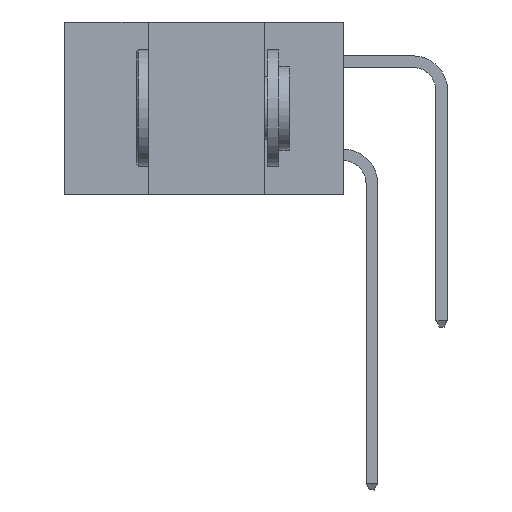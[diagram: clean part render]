
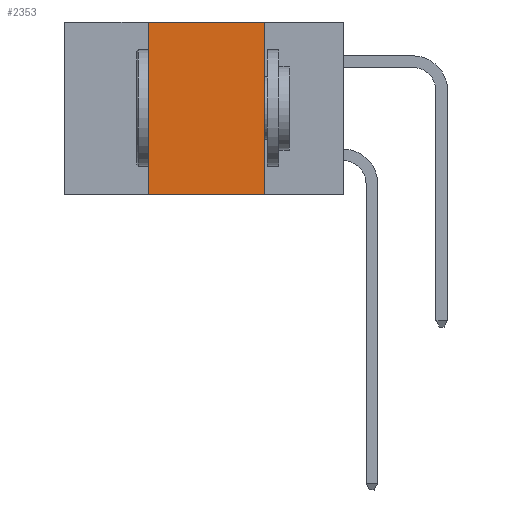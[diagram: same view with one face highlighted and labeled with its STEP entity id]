
A CAD part, left-side view. The second image highlights one B-rep face of the part: STEP entity #2353.
In plain terms, the highlighted planar face has unit normal (-1, 0, 0).
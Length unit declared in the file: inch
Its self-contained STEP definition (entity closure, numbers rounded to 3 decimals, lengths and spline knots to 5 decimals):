
#746 = VECTOR ( 'NONE', #16608, 39.37008 ) ;
#815 = CARTESIAN_POINT ( 'NONE',  ( 0., 0.6, 0. ) ) ;
#844 = CARTESIAN_POINT ( 'NONE',  ( 0., 0.17, 0. ) ) ;
#1459 = ORIENTED_EDGE ( 'NONE', *, *, #2229, .T. ) ;
#2229 = EDGE_CURVE ( 'NONE', #6645, #19244, #9526, .T. ) ;
#2277 = PLANE ( 'NONE',  #7809 ) ;
#2353 = ADVANCED_FACE ( 'NONE', ( #14612 ), #2277, .F. ) ;
#2810 = DIRECTION ( 'NONE',  ( 0., -1., 0. ) ) ;
#3383 = CARTESIAN_POINT ( 'NONE',  ( 0., 0.17, 0. ) ) ;
#3513 = CARTESIAN_POINT ( 'NONE',  ( 0., 0.42, 0. ) ) ;
#4089 = ORIENTED_EDGE ( 'NONE', *, *, #16455, .F. ) ;
#4369 = DIRECTION ( 'NONE',  ( 1., 0., 0. ) ) ;
#6614 = DIRECTION ( 'NONE',  ( 0., 0., 1. ) ) ;
#6645 = VERTEX_POINT ( 'NONE', #18023 ) ;
#7809 = AXIS2_PLACEMENT_3D ( 'NONE', #815, #4369, #8107 ) ;
#8107 = DIRECTION ( 'NONE',  ( 0., 0., -1. ) ) ;
#8131 = DIRECTION ( 'NONE',  ( 0., 0., -1. ) ) ;
#9526 = LINE ( 'NONE', #19533, #746 ) ;
#10355 = VECTOR ( 'NONE', #2810, 39.37008 ) ;
#11528 = EDGE_LOOP ( 'NONE', ( #15240, #4089, #16636, #1459 ) ) ;
#13501 = LINE ( 'NONE', #15621, #17454 ) ;
#14286 = LINE ( 'NONE', #14978, #10355 ) ;
#14298 = VERTEX_POINT ( 'NONE', #3513 ) ;
#14612 = FACE_OUTER_BOUND ( 'NONE', #11528, .T. ) ;
#14872 = EDGE_CURVE ( 'NONE', #15494, #19244, #15067, .T. ) ;
#14978 = CARTESIAN_POINT ( 'NONE',  ( 0., 0.6, 0. ) ) ;
#15067 = LINE ( 'NONE', #3383, #18568 ) ;
#15240 = ORIENTED_EDGE ( 'NONE', *, *, #14872, .F. ) ;
#15494 = VERTEX_POINT ( 'NONE', #844 ) ;
#15621 = CARTESIAN_POINT ( 'NONE',  ( 0., 0.42, 0. ) ) ;
#16455 = EDGE_CURVE ( 'NONE', #14298, #15494, #14286, .T. ) ;
#16608 = DIRECTION ( 'NONE',  ( 0., -1., 0. ) ) ;
#16636 = ORIENTED_EDGE ( 'NONE', *, *, #18844, .F. ) ;
#17454 = VECTOR ( 'NONE', #6614, 39.37008 ) ;
#18023 = CARTESIAN_POINT ( 'NONE',  ( 0., 0.42, -0.37 ) ) ;
#18568 = VECTOR ( 'NONE', #8131, 39.37008 ) ;
#18844 = EDGE_CURVE ( 'NONE', #6645, #14298, #13501, .T. ) ;
#19244 = VERTEX_POINT ( 'NONE', #19559 ) ;
#19533 = CARTESIAN_POINT ( 'NONE',  ( 0., 0.6, -0.37 ) ) ;
#19559 = CARTESIAN_POINT ( 'NONE',  ( 0., 0.17, -0.37 ) ) ;
